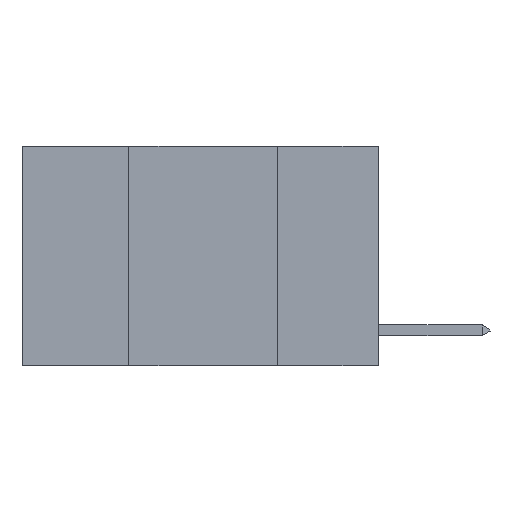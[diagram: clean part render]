
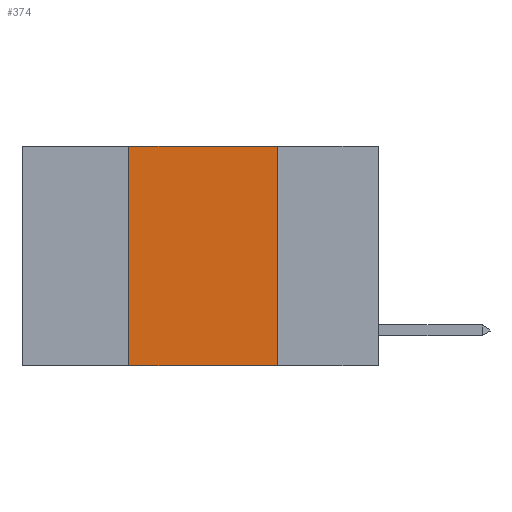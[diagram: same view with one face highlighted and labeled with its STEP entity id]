
A CAD part, left-side view. The second image highlights one B-rep face of the part: STEP entity #374.
In plain terms, the highlighted planar face has unit normal (-1, 0, 0).
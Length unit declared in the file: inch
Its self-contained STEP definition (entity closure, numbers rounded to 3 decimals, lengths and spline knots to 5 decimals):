
#293 = CARTESIAN_POINT ( 'NONE',  ( 0., 0.17, 0. ) ) ;
#374 = ADVANCED_FACE ( 'NONE', ( #1282 ), #2084, .F. ) ;
#1159 = LINE ( 'NONE', #4446, #6150 ) ;
#1282 = FACE_OUTER_BOUND ( 'NONE', #8776, .T. ) ;
#1393 = DIRECTION ( 'NONE',  ( 0., 0., -1. ) ) ;
#1428 = DIRECTION ( 'NONE',  ( 1., 0., 0. ) ) ;
#1468 = CARTESIAN_POINT ( 'NONE',  ( 0., 0.6, 0. ) ) ;
#2084 = PLANE ( 'NONE',  #2357 ) ;
#2357 = AXIS2_PLACEMENT_3D ( 'NONE', #1468, #1428, #1393 ) ;
#2394 = VERTEX_POINT ( 'NONE', #9022 ) ;
#2756 = VERTEX_POINT ( 'NONE', #14053 ) ;
#2890 = VECTOR ( 'NONE', #13097, 39.37008 ) ;
#2998 = ORIENTED_EDGE ( 'NONE', *, *, #10786, .T. ) ;
#3368 = VECTOR ( 'NONE', #11475, 39.37008 ) ;
#4072 = LINE ( 'NONE', #293, #3368 ) ;
#4446 = CARTESIAN_POINT ( 'NONE',  ( 0., 0.6, -0.37 ) ) ;
#4565 = ORIENTED_EDGE ( 'NONE', *, *, #12961, .F. ) ;
#4739 = VERTEX_POINT ( 'NONE', #11375 ) ;
#5083 = CARTESIAN_POINT ( 'NONE',  ( 0., 0.6, 0. ) ) ;
#6150 = VECTOR ( 'NONE', #11067, 39.37008 ) ;
#7650 = CARTESIAN_POINT ( 'NONE',  ( 0., 0.42, 0. ) ) ;
#8776 = EDGE_LOOP ( 'NONE', ( #4565, #10599, #10054, #2998 ) ) ;
#8779 = LINE ( 'NONE', #11998, #2890 ) ;
#9022 = CARTESIAN_POINT ( 'NONE',  ( 0., 0.17, 0. ) ) ;
#10054 = ORIENTED_EDGE ( 'NONE', *, *, #11494, .F. ) ;
#10475 = VECTOR ( 'NONE', #11720, 39.37008 ) ;
#10599 = ORIENTED_EDGE ( 'NONE', *, *, #13146, .F. ) ;
#10786 = EDGE_CURVE ( 'NONE', #4739, #2756, #1159, .T. ) ;
#11067 = DIRECTION ( 'NONE',  ( 0., -1., 0. ) ) ;
#11375 = CARTESIAN_POINT ( 'NONE',  ( 0., 0.42, -0.37 ) ) ;
#11475 = DIRECTION ( 'NONE',  ( 0., 0., -1. ) ) ;
#11494 = EDGE_CURVE ( 'NONE', #4739, #12041, #8779, .T. ) ;
#11720 = DIRECTION ( 'NONE',  ( 0., -1., 0. ) ) ;
#11998 = CARTESIAN_POINT ( 'NONE',  ( 0., 0.42, 0. ) ) ;
#12041 = VERTEX_POINT ( 'NONE', #7650 ) ;
#12961 = EDGE_CURVE ( 'NONE', #2394, #2756, #4072, .T. ) ;
#13025 = LINE ( 'NONE', #5083, #10475 ) ;
#13097 = DIRECTION ( 'NONE',  ( 0., 0., 1. ) ) ;
#13146 = EDGE_CURVE ( 'NONE', #12041, #2394, #13025, .T. ) ;
#14053 = CARTESIAN_POINT ( 'NONE',  ( 0., 0.17, -0.37 ) ) ;
